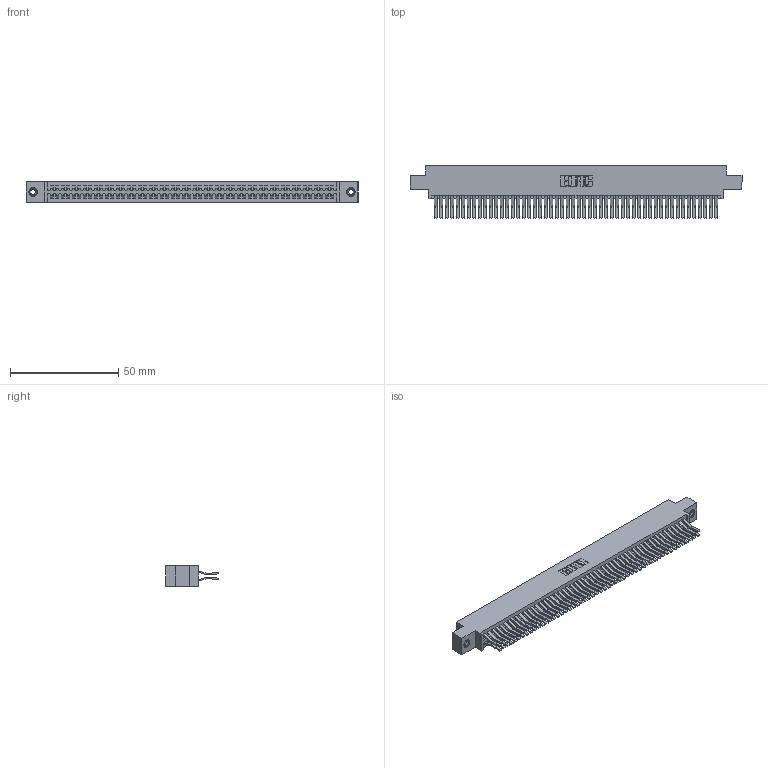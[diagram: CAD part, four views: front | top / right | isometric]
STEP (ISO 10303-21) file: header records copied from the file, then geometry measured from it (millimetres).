
FILE_DESCRIPTION (( 'STEP AP203' ), '1' );
FILE_NAME ('345-104-560-808.STEP', '2018-10-06T02:17:42', ( '' ), ( '' ), 'SwSTEP 2.0', 'SolidWorks 2016', '' );
FILE_SCHEMA (( 'CONFIG_CONTROL_DESIGN' ));
Length unit declared in the file: inch
Products named in the file (4): 345-292-001_560 Tail; 345-104-560-808; 345 Part_0.170 Offset - 0.156 Dia-TI; 345-250-001_345-250-003-102
Assembly tree (107 placements, depth 2):
  345-104-560-808
    345 Part_0.170 Offset - 0.156 Dia-TI
    345-292-001_560 Tail  x104
    345-250-001_345-250-003-102  x2
Bounding box: 153.29 x 24.45 x 9.4 mm (x, y, z)
Volume: 15545.3 mm3; surface area: 25082.3 mm2
Topology: 107 solids, 107 shells, 5598 faces, 16609 edges, 10926 vertices
Faces by surface type: plane 3548, cylinder 2034, cone 12, torus 4
Entity records: 40860 total; most frequent: CARTESIAN_POINT 6823, ORIENTED_EDGE 6750, DIRECTION 6033, EDGE_CURVE 3375, LINE 3011, VECTOR 3011, VERTEX_POINT 2244, AXIS2_PLACEMENT_3D 1511
